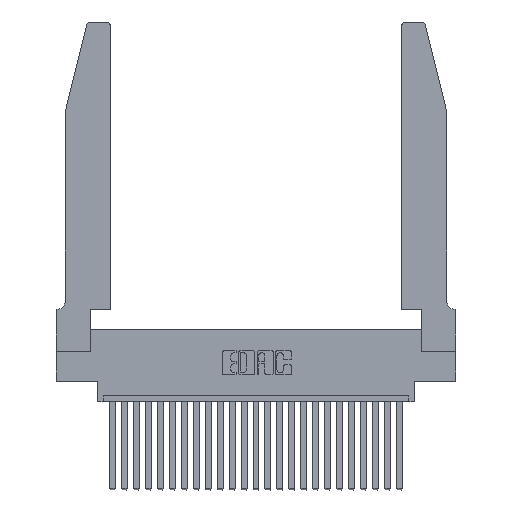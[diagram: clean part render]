
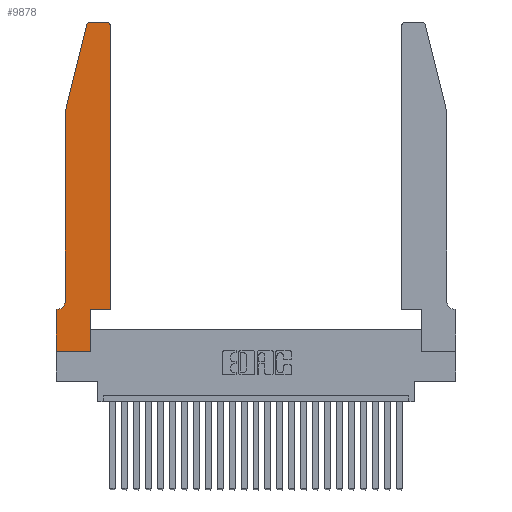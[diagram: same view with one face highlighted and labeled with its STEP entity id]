
A CAD part, top view. The second image highlights one B-rep face of the part: STEP entity #9878.
In plain terms, the highlighted planar face has unit normal (0, 0, 1).
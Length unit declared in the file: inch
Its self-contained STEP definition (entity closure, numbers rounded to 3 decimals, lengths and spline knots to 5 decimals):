
#131 = LINE ( 'NONE', #14307, #24141 ) ;
#189 = VERTEX_POINT ( 'NONE', #1427 ) ;
#389 = LINE ( 'NONE', #3409, #20996 ) ;
#625 = EDGE_CURVE ( 'NONE', #2363, #23208, #8864, .T. ) ;
#994 = CARTESIAN_POINT ( 'NONE',  ( 0., 0.35, 0.37 ) ) ;
#1111 = CARTESIAN_POINT ( 'NONE',  ( 0.4505, 0.35, 0.37 ) ) ;
#1427 = CARTESIAN_POINT ( 'NONE',  ( 0., 0., 0.37 ) ) ;
#1561 = DIRECTION ( 'NONE',  ( 1., 0., 0. ) ) ;
#2130 = LINE ( 'NONE', #18641, #24943 ) ;
#2363 = VERTEX_POINT ( 'NONE', #4026 ) ;
#2390 = CARTESIAN_POINT ( 'NONE',  ( 0.0755, 2., 0.37 ) ) ;
#2655 = DIRECTION ( 'NONE',  ( 1., 0., 0. ) ) ;
#3021 = EDGE_CURVE ( 'NONE', #23617, #2363, #2130, .T. ) ;
#3101 = ORIENTED_EDGE ( 'NONE', *, *, #15747, .T. ) ;
#3228 = LINE ( 'NONE', #18886, #8889 ) ;
#3250 = ORIENTED_EDGE ( 'NONE', *, *, #15500, .T. ) ;
#3409 = CARTESIAN_POINT ( 'NONE',  ( 0.2865, 0.35, 0.37 ) ) ;
#3625 = VECTOR ( 'NONE', #4104, 39.37008 ) ;
#3930 = CIRCLE ( 'NONE', #18112, 0.03 ) ;
#4026 = CARTESIAN_POINT ( 'NONE',  ( 0.4505, 2.72, 0.37 ) ) ;
#4032 = CIRCLE ( 'NONE', #6634, 0.07 ) ;
#4104 = DIRECTION ( 'NONE',  ( -1., 0., 0. ) ) ;
#4308 = ORIENTED_EDGE ( 'NONE', *, *, #24122, .T. ) ;
#5328 = ORIENTED_EDGE ( 'NONE', *, *, #13248, .T. ) ;
#5431 = EDGE_CURVE ( 'NONE', #8583, #19142, #3228, .T. ) ;
#6232 = VERTEX_POINT ( 'NONE', #6725 ) ;
#6533 = CARTESIAN_POINT ( 'NONE',  ( 0.4205, 2.72, 0.37 ) ) ;
#6572 = LINE ( 'NONE', #9892, #16574 ) ;
#6634 = AXIS2_PLACEMENT_3D ( 'NONE', #13753, #15048, #11470 ) ;
#6712 = LINE ( 'NONE', #17500, #16067 ) ;
#6725 = CARTESIAN_POINT ( 'NONE',  ( 0.0055, 0.35, 0.37 ) ) ;
#6801 = DIRECTION ( 'NONE',  ( 0., 0., 1. ) ) ;
#6894 = VERTEX_POINT ( 'NONE', #7286 ) ;
#7110 = LINE ( 'NONE', #9227, #9896 ) ;
#7233 = CARTESIAN_POINT ( 'NONE',  ( 0.25487, 2.72718, 0.37 ) ) ;
#7286 = CARTESIAN_POINT ( 'NONE',  ( 0.2865, 0.35, 0.37 ) ) ;
#7485 = DIRECTION ( 'NONE',  ( 0., -1., 0. ) ) ;
#7679 = VERTEX_POINT ( 'NONE', #14315 ) ;
#8147 = LINE ( 'NONE', #8412, #17206 ) ;
#8412 = CARTESIAN_POINT ( 'NONE',  ( 0.4505, 0.35, 0.37 ) ) ;
#8583 = VERTEX_POINT ( 'NONE', #7233 ) ;
#8864 = CIRCLE ( 'NONE', #12141, 0.03 ) ;
#8889 = VECTOR ( 'NONE', #22684, 39.37008 ) ;
#9162 = ORIENTED_EDGE ( 'NONE', *, *, #12098, .T. ) ;
#9227 = CARTESIAN_POINT ( 'NONE',  ( 0., 0., 0.37 ) ) ;
#9326 = ORIENTED_EDGE ( 'NONE', *, *, #20894, .T. ) ;
#9878 = ADVANCED_FACE ( 'NONE', ( #19553 ), #12314, .T. ) ;
#9892 = CARTESIAN_POINT ( 'NONE',  ( 0., 0., 0.37 ) ) ;
#9896 = VECTOR ( 'NONE', #1561, 39.37008 ) ;
#9957 = EDGE_CURVE ( 'NONE', #6232, #14448, #10188, .T. ) ;
#10188 = LINE ( 'NONE', #24147, #3625 ) ;
#10341 = DIRECTION ( 'NONE',  ( 0., 0., 1. ) ) ;
#11060 = EDGE_LOOP ( 'NONE', ( #9162, #4308, #15161, #5328, #3250, #16216, #15584, #9326, #12713, #3101, #12964, #23212 ) ) ;
#11422 = CARTESIAN_POINT ( 'NONE',  ( 0.0755, 0.42, 0.37 ) ) ;
#11470 = DIRECTION ( 'NONE',  ( -1., 0., 0. ) ) ;
#12050 = DIRECTION ( 'NONE',  ( 1., 0., 0. ) ) ;
#12098 = EDGE_CURVE ( 'NONE', #23208, #19645, #131, .T. ) ;
#12141 = AXIS2_PLACEMENT_3D ( 'NONE', #6533, #6801, #2655 ) ;
#12220 = CARTESIAN_POINT ( 'NONE',  ( 0., 0.35, 0.37 ) ) ;
#12314 = PLANE ( 'NONE',  #12570 ) ;
#12570 = AXIS2_PLACEMENT_3D ( 'NONE', #12220, #22367, #12050 ) ;
#12713 = ORIENTED_EDGE ( 'NONE', *, *, #23254, .T. ) ;
#12964 = ORIENTED_EDGE ( 'NONE', *, *, #3021, .T. ) ;
#13248 = EDGE_CURVE ( 'NONE', #19142, #24389, #6712, .T. ) ;
#13753 = CARTESIAN_POINT ( 'NONE',  ( 0.0055, 0.42, 0.37 ) ) ;
#14130 = DIRECTION ( 'NONE',  ( -1., 0., 0. ) ) ;
#14307 = CARTESIAN_POINT ( 'NONE',  ( 0.2605, 2.75, 0.37 ) ) ;
#14315 = CARTESIAN_POINT ( 'NONE',  ( 0.2865, 0., 0.37 ) ) ;
#14448 = VERTEX_POINT ( 'NONE', #994 ) ;
#14796 = CARTESIAN_POINT ( 'NONE',  ( 0.4205, 2.75, 0.37 ) ) ;
#15048 = DIRECTION ( 'NONE',  ( 0., 0., -1. ) ) ;
#15161 = ORIENTED_EDGE ( 'NONE', *, *, #5431, .T. ) ;
#15500 = EDGE_CURVE ( 'NONE', #24389, #6232, #4032, .T. ) ;
#15584 = ORIENTED_EDGE ( 'NONE', *, *, #18161, .T. ) ;
#15747 = EDGE_CURVE ( 'NONE', #6894, #23617, #8147, .T. ) ;
#16067 = VECTOR ( 'NONE', #7485, 39.37008 ) ;
#16216 = ORIENTED_EDGE ( 'NONE', *, *, #9957, .T. ) ;
#16574 = VECTOR ( 'NONE', #21719, 39.37008 ) ;
#16846 = DIRECTION ( 'NONE',  ( 0., 1., 0. ) ) ;
#17037 = CARTESIAN_POINT ( 'NONE',  ( 0.284, 2.75, 0.37 ) ) ;
#17206 = VECTOR ( 'NONE', #22729, 39.37008 ) ;
#17500 = CARTESIAN_POINT ( 'NONE',  ( 0.0755, 2., 0.37 ) ) ;
#18112 = AXIS2_PLACEMENT_3D ( 'NONE', #18271, #10341, #20549 ) ;
#18161 = EDGE_CURVE ( 'NONE', #14448, #189, #6572, .T. ) ;
#18271 = CARTESIAN_POINT ( 'NONE',  ( 0.284, 2.72, 0.37 ) ) ;
#18641 = CARTESIAN_POINT ( 'NONE',  ( 0.4505, 0.35, 0.37 ) ) ;
#18886 = CARTESIAN_POINT ( 'NONE',  ( 0.0755, 2., 0.37 ) ) ;
#19142 = VERTEX_POINT ( 'NONE', #2390 ) ;
#19553 = FACE_OUTER_BOUND ( 'NONE', #11060, .T. ) ;
#19645 = VERTEX_POINT ( 'NONE', #17037 ) ;
#20549 = DIRECTION ( 'NONE',  ( 1., 0., 0. ) ) ;
#20894 = EDGE_CURVE ( 'NONE', #189, #7679, #7110, .T. ) ;
#20996 = VECTOR ( 'NONE', #23189, 39.37008 ) ;
#21719 = DIRECTION ( 'NONE',  ( 0., -1., 0. ) ) ;
#22367 = DIRECTION ( 'NONE',  ( 0., 0., 1. ) ) ;
#22684 = DIRECTION ( 'NONE',  ( -0.239, -0.971, 0. ) ) ;
#22729 = DIRECTION ( 'NONE',  ( 1., 0., 0. ) ) ;
#23189 = DIRECTION ( 'NONE',  ( 0., 1., 0. ) ) ;
#23208 = VERTEX_POINT ( 'NONE', #14796 ) ;
#23212 = ORIENTED_EDGE ( 'NONE', *, *, #625, .T. ) ;
#23254 = EDGE_CURVE ( 'NONE', #7679, #6894, #389, .T. ) ;
#23617 = VERTEX_POINT ( 'NONE', #1111 ) ;
#24122 = EDGE_CURVE ( 'NONE', #19645, #8583, #3930, .T. ) ;
#24141 = VECTOR ( 'NONE', #14130, 39.37008 ) ;
#24147 = CARTESIAN_POINT ( 'NONE',  ( 0.0755, 0.35, 0.37 ) ) ;
#24389 = VERTEX_POINT ( 'NONE', #11422 ) ;
#24943 = VECTOR ( 'NONE', #16846, 39.37008 ) ;
